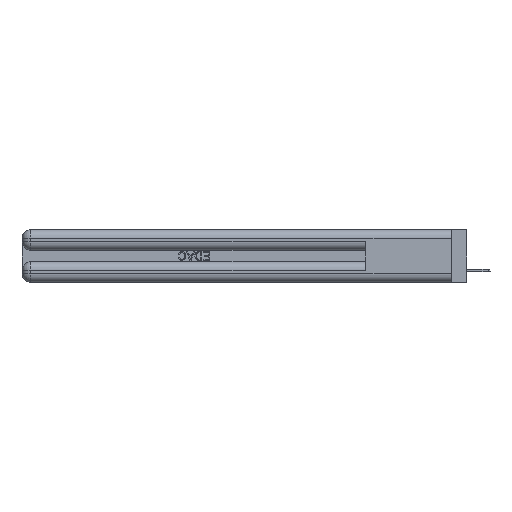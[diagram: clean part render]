
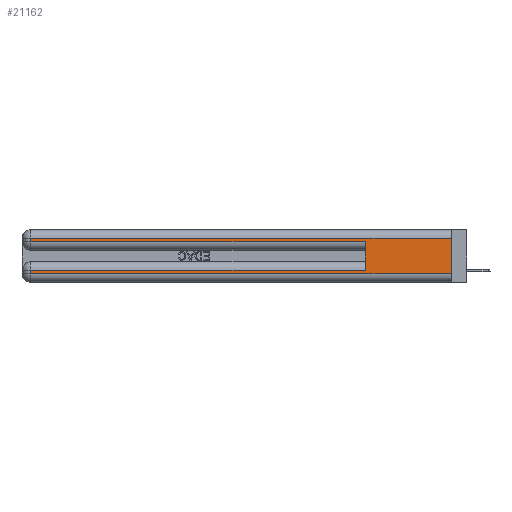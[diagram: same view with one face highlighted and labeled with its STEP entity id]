
A CAD part, left-side view. The second image highlights one B-rep face of the part: STEP entity #21162.
In plain terms, the highlighted planar face has unit normal (-1, 0, 0).
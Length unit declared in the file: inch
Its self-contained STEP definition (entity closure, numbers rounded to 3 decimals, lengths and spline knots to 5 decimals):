
#31 = CARTESIAN_POINT ( 'NONE',  ( 0., 0., 0.285 ) ) ;
#321 = DIRECTION ( 'NONE',  ( 0., -1., 0. ) ) ;
#2085 = VECTOR ( 'NONE', #17515, 39.37008 ) ;
#2814 = ORIENTED_EDGE ( 'NONE', *, *, #44721, .T. ) ;
#3010 = ORIENTED_EDGE ( 'NONE', *, *, #5992, .F. ) ;
#3198 = EDGE_CURVE ( 'NONE', #21423, #27673, #39257, .T. ) ;
#3911 = LINE ( 'NONE', #12228, #15696 ) ;
#4686 = FACE_OUTER_BOUND ( 'NONE', #14659, .T. ) ;
#4736 = CARTESIAN_POINT ( 'NONE',  ( 0., 2.94, 0.085 ) ) ;
#5729 = VECTOR ( 'NONE', #21204, 39.37008 ) ;
#5936 = ORIENTED_EDGE ( 'NONE', *, *, #39079, .T. ) ;
#5992 = EDGE_CURVE ( 'NONE', #9385, #27673, #11559, .T. ) ;
#6609 = LINE ( 'NONE', #42049, #32283 ) ;
#9385 = VERTEX_POINT ( 'NONE', #35022 ) ;
#10178 = VERTEX_POINT ( 'NONE', #31325 ) ;
#10772 = VECTOR ( 'NONE', #321, 39.37008 ) ;
#11559 = LINE ( 'NONE', #25792, #16073 ) ;
#12228 = CARTESIAN_POINT ( 'NONE',  ( 0., 0., 0.085 ) ) ;
#12370 = CARTESIAN_POINT ( 'NONE',  ( 0., 0., 0.31 ) ) ;
#12545 = DIRECTION ( 'NONE',  ( 0., 1., 0. ) ) ;
#13777 = CARTESIAN_POINT ( 'NONE',  ( 0., 0., 0.37 ) ) ;
#14321 = VERTEX_POINT ( 'NONE', #22500 ) ;
#14659 = EDGE_LOOP ( 'NONE', ( #18752, #5936, #16799, #39853, #3010, #30907, #24903, #2814 ) ) ;
#14945 = PLANE ( 'NONE',  #20860 ) ;
#15273 = DIRECTION ( 'NONE',  ( 1., 0., 0. ) ) ;
#15279 = CARTESIAN_POINT ( 'NONE',  ( 0., 2.94, 0.285 ) ) ;
#15696 = VECTOR ( 'NONE', #12545, 39.37008 ) ;
#15869 = VECTOR ( 'NONE', #18788, 39.37008 ) ;
#15912 = EDGE_CURVE ( 'NONE', #32057, #14321, #43739, .T. ) ;
#16073 = VECTOR ( 'NONE', #29536, 39.37008 ) ;
#16799 = ORIENTED_EDGE ( 'NONE', *, *, #40337, .T. ) ;
#17515 = DIRECTION ( 'NONE',  ( 0., -1., 0. ) ) ;
#17615 = CARTESIAN_POINT ( 'NONE',  ( 0., 2.94, 0.37 ) ) ;
#18752 = ORIENTED_EDGE ( 'NONE', *, *, #34012, .F. ) ;
#18788 = DIRECTION ( 'NONE',  ( 0., 0., -1. ) ) ;
#20860 = AXIS2_PLACEMENT_3D ( 'NONE', #36672, #15273, #25296 ) ;
#21162 = ADVANCED_FACE ( 'NONE', ( #4686 ), #14945, .F. ) ;
#21204 = DIRECTION ( 'NONE',  ( 0., 0., -1. ) ) ;
#21423 = VERTEX_POINT ( 'NONE', #15279 ) ;
#22500 = CARTESIAN_POINT ( 'NONE',  ( 0., 2.94, 0.06 ) ) ;
#23334 = DIRECTION ( 'NONE',  ( 0., 1., 0. ) ) ;
#24903 = ORIENTED_EDGE ( 'NONE', *, *, #15912, .T. ) ;
#25296 = DIRECTION ( 'NONE',  ( 0., 0., -1. ) ) ;
#25792 = CARTESIAN_POINT ( 'NONE',  ( 0., 0.6, 0.145 ) ) ;
#26413 = CARTESIAN_POINT ( 'NONE',  ( 0., 0., 0.06 ) ) ;
#27673 = VERTEX_POINT ( 'NONE', #38479 ) ;
#28918 = LINE ( 'NONE', #35464, #2085 ) ;
#29536 = DIRECTION ( 'NONE',  ( 0., 0., 1. ) ) ;
#30648 = EDGE_CURVE ( 'NONE', #9385, #32057, #3911, .T. ) ;
#30907 = ORIENTED_EDGE ( 'NONE', *, *, #30648, .T. ) ;
#31325 = CARTESIAN_POINT ( 'NONE',  ( 0., 0., 0.31 ) ) ;
#31588 = DIRECTION ( 'NONE',  ( 0., 0., -1. ) ) ;
#31906 = VERTEX_POINT ( 'NONE', #39416 ) ;
#32057 = VERTEX_POINT ( 'NONE', #4736 ) ;
#32283 = VECTOR ( 'NONE', #31588, 39.37008 ) ;
#34012 = EDGE_CURVE ( 'NONE', #10178, #44793, #46057, .T. ) ;
#35022 = CARTESIAN_POINT ( 'NONE',  ( 0., 0.6, 0.085 ) ) ;
#35175 = VECTOR ( 'NONE', #23334, 39.37008 ) ;
#35464 = CARTESIAN_POINT ( 'NONE',  ( 0., 0., 0.06 ) ) ;
#36672 = CARTESIAN_POINT ( 'NONE',  ( 0., 0., 0.37 ) ) ;
#38479 = CARTESIAN_POINT ( 'NONE',  ( 0., 0.6, 0.285 ) ) ;
#39055 = LINE ( 'NONE', #12370, #35175 ) ;
#39079 = EDGE_CURVE ( 'NONE', #10178, #31906, #39055, .T. ) ;
#39257 = LINE ( 'NONE', #31, #10772 ) ;
#39416 = CARTESIAN_POINT ( 'NONE',  ( 0., 2.94, 0.31 ) ) ;
#39853 = ORIENTED_EDGE ( 'NONE', *, *, #3198, .T. ) ;
#40337 = EDGE_CURVE ( 'NONE', #31906, #21423, #6609, .T. ) ;
#42049 = CARTESIAN_POINT ( 'NONE',  ( 0., 2.94, 0.37 ) ) ;
#43739 = LINE ( 'NONE', #17615, #5729 ) ;
#44721 = EDGE_CURVE ( 'NONE', #14321, #44793, #28918, .T. ) ;
#44793 = VERTEX_POINT ( 'NONE', #26413 ) ;
#46057 = LINE ( 'NONE', #13777, #15869 ) ;
